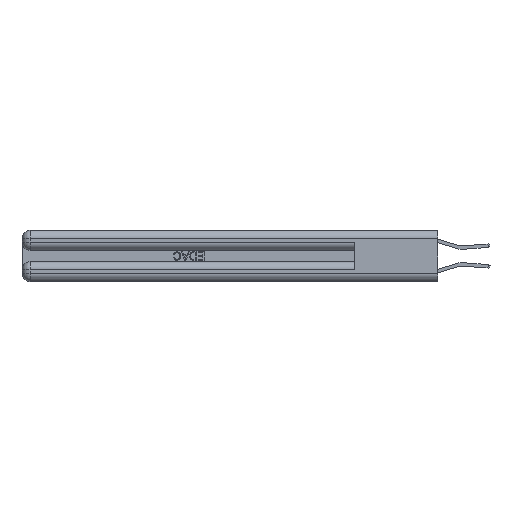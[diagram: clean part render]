
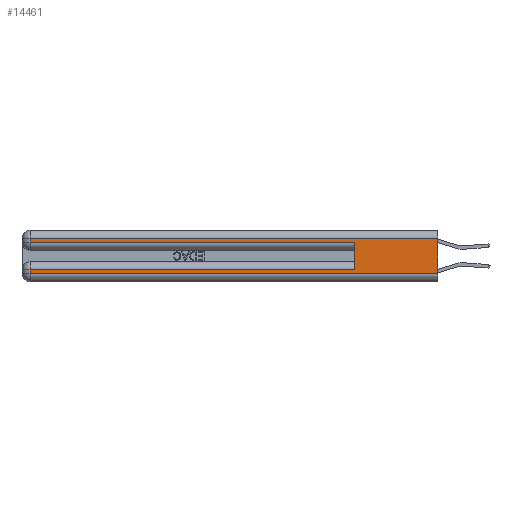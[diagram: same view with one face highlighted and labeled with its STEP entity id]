
A CAD part, left-side view. The second image highlights one B-rep face of the part: STEP entity #14461.
In plain terms, the highlighted planar face has unit normal (-1, 0, 0).
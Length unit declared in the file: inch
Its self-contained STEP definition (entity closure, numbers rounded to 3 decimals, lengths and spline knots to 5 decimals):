
#177 = LINE ( 'NONE', #22594, #34742 ) ;
#820 = LINE ( 'NONE', #32366, #24215 ) ;
#936 = VERTEX_POINT ( 'NONE', #26436 ) ;
#983 = DIRECTION ( 'NONE',  ( 0., 1., 0. ) ) ;
#1390 = EDGE_CURVE ( 'NONE', #32221, #20741, #19556, .T. ) ;
#1423 = EDGE_CURVE ( 'NONE', #17106, #10376, #820, .T. ) ;
#2087 = EDGE_CURVE ( 'NONE', #8926, #7866, #24603, .T. ) ;
#2161 = EDGE_CURVE ( 'NONE', #936, #7866, #20789, .T. ) ;
#3198 = CARTESIAN_POINT ( 'NONE',  ( 0., 0., 0.37 ) ) ;
#3286 = CARTESIAN_POINT ( 'NONE',  ( 0., 0.6, 0.145 ) ) ;
#3780 = EDGE_CURVE ( 'NONE', #5973, #32221, #25353, .T. ) ;
#4046 = ORIENTED_EDGE ( 'NONE', *, *, #1390, .T. ) ;
#4447 = LINE ( 'NONE', #30751, #18482 ) ;
#4887 = CARTESIAN_POINT ( 'NONE',  ( 0., 0., 0.285 ) ) ;
#5552 = CARTESIAN_POINT ( 'NONE',  ( 0., 2.94, 0.31 ) ) ;
#5973 = VERTEX_POINT ( 'NONE', #26931 ) ;
#6433 = ORIENTED_EDGE ( 'NONE', *, *, #2161, .F. ) ;
#6951 = ORIENTED_EDGE ( 'NONE', *, *, #1423, .T. ) ;
#7379 = FACE_OUTER_BOUND ( 'NONE', #11584, .T. ) ;
#7866 = VERTEX_POINT ( 'NONE', #27870 ) ;
#8926 = VERTEX_POINT ( 'NONE', #15258 ) ;
#9805 = ORIENTED_EDGE ( 'NONE', *, *, #3780, .T. ) ;
#10045 = VECTOR ( 'NONE', #12064, 39.37008 ) ;
#10275 = AXIS2_PLACEMENT_3D ( 'NONE', #30956, #14609, #28004 ) ;
#10376 = VERTEX_POINT ( 'NONE', #5552 ) ;
#10653 = DIRECTION ( 'NONE',  ( 0., 1., 0. ) ) ;
#11584 = EDGE_LOOP ( 'NONE', ( #30961, #6951, #13369, #30558, #6433, #16891, #9805, #4046 ) ) ;
#11598 = CARTESIAN_POINT ( 'NONE',  ( 0., 2.94, 0.06 ) ) ;
#11797 = DIRECTION ( 'NONE',  ( 0., 0., -1. ) ) ;
#12064 = DIRECTION ( 'NONE',  ( 0., 0., -1. ) ) ;
#13369 = ORIENTED_EDGE ( 'NONE', *, *, #27027, .T. ) ;
#13508 = LINE ( 'NONE', #3198, #28467 ) ;
#14229 = DIRECTION ( 'NONE',  ( 0., 0., 1. ) ) ;
#14461 = ADVANCED_FACE ( 'NONE', ( #7379 ), #17121, .F. ) ;
#14609 = DIRECTION ( 'NONE',  ( 1., 0., 0. ) ) ;
#14809 = VECTOR ( 'NONE', #14229, 39.37008 ) ;
#15258 = CARTESIAN_POINT ( 'NONE',  ( 0., 2.94, 0.285 ) ) ;
#16891 = ORIENTED_EDGE ( 'NONE', *, *, #27093, .T. ) ;
#17106 = VERTEX_POINT ( 'NONE', #19348 ) ;
#17121 = PLANE ( 'NONE',  #10275 ) ;
#17384 = VECTOR ( 'NONE', #35153, 39.37008 ) ;
#18482 = VECTOR ( 'NONE', #983, 39.37008 ) ;
#18959 = EDGE_CURVE ( 'NONE', #17106, #20741, #13508, .T. ) ;
#19348 = CARTESIAN_POINT ( 'NONE',  ( 0., 0., 0.31 ) ) ;
#19556 = LINE ( 'NONE', #32131, #29805 ) ;
#19711 = CARTESIAN_POINT ( 'NONE',  ( 0., 0., 0.06 ) ) ;
#20741 = VERTEX_POINT ( 'NONE', #19711 ) ;
#20789 = LINE ( 'NONE', #3286, #14809 ) ;
#22594 = CARTESIAN_POINT ( 'NONE',  ( 0., 2.94, 0.37 ) ) ;
#24215 = VECTOR ( 'NONE', #10653, 39.37008 ) ;
#24603 = LINE ( 'NONE', #4887, #17384 ) ;
#25353 = LINE ( 'NONE', #30788, #10045 ) ;
#26436 = CARTESIAN_POINT ( 'NONE',  ( 0., 0.6, 0.085 ) ) ;
#26931 = CARTESIAN_POINT ( 'NONE',  ( 0., 2.94, 0.085 ) ) ;
#27027 = EDGE_CURVE ( 'NONE', #10376, #8926, #177, .T. ) ;
#27093 = EDGE_CURVE ( 'NONE', #936, #5973, #4447, .T. ) ;
#27766 = DIRECTION ( 'NONE',  ( 0., 0., -1. ) ) ;
#27870 = CARTESIAN_POINT ( 'NONE',  ( 0., 0.6, 0.285 ) ) ;
#28004 = DIRECTION ( 'NONE',  ( 0., 0., -1. ) ) ;
#28467 = VECTOR ( 'NONE', #27766, 39.37008 ) ;
#29741 = DIRECTION ( 'NONE',  ( 0., -1., 0. ) ) ;
#29805 = VECTOR ( 'NONE', #29741, 39.37008 ) ;
#30558 = ORIENTED_EDGE ( 'NONE', *, *, #2087, .T. ) ;
#30751 = CARTESIAN_POINT ( 'NONE',  ( 0., 0., 0.085 ) ) ;
#30788 = CARTESIAN_POINT ( 'NONE',  ( 0., 2.94, 0.37 ) ) ;
#30956 = CARTESIAN_POINT ( 'NONE',  ( 0., 0., 0.37 ) ) ;
#30961 = ORIENTED_EDGE ( 'NONE', *, *, #18959, .F. ) ;
#32131 = CARTESIAN_POINT ( 'NONE',  ( 0., 0., 0.06 ) ) ;
#32221 = VERTEX_POINT ( 'NONE', #11598 ) ;
#32366 = CARTESIAN_POINT ( 'NONE',  ( 0., 0., 0.31 ) ) ;
#34742 = VECTOR ( 'NONE', #11797, 39.37008 ) ;
#35153 = DIRECTION ( 'NONE',  ( 0., -1., 0. ) ) ;
